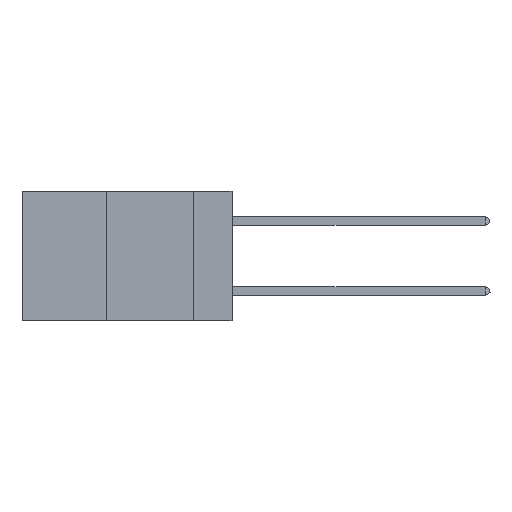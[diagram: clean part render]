
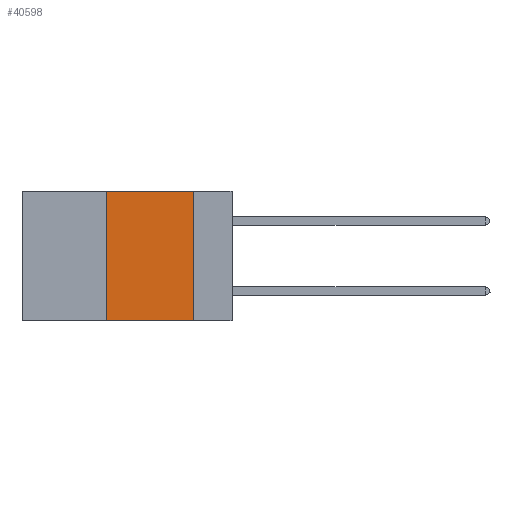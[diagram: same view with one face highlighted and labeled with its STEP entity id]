
A CAD part, left-side view. The second image highlights one B-rep face of the part: STEP entity #40598.
In plain terms, the highlighted planar face has unit normal (-1, 0, 0).
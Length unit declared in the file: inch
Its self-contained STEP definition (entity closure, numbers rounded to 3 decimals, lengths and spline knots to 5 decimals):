
#382 = CARTESIAN_POINT ( 'NONE',  ( 0., 0.36, 0. ) ) ;
#1065 = VECTOR ( 'NONE', #1527, 39.37008 ) ;
#1527 = DIRECTION ( 'NONE',  ( 0., -1., 0. ) ) ;
#1857 = PLANE ( 'NONE',  #9017 ) ;
#2137 = VECTOR ( 'NONE', #36991, 39.37008 ) ;
#2218 = FACE_OUTER_BOUND ( 'NONE', #4220, .T. ) ;
#4220 = EDGE_LOOP ( 'NONE', ( #26346, #16620, #9751, #11718 ) ) ;
#6158 = EDGE_CURVE ( 'NONE', #21618, #41178, #9960, .T. ) ;
#6768 = CARTESIAN_POINT ( 'NONE',  ( 0., 0.6, -0.37 ) ) ;
#8597 = CARTESIAN_POINT ( 'NONE',  ( 0., 0.36, -0.37 ) ) ;
#9017 = AXIS2_PLACEMENT_3D ( 'NONE', #24140, #38296, #34073 ) ;
#9751 = ORIENTED_EDGE ( 'NONE', *, *, #23427, .F. ) ;
#9761 = CARTESIAN_POINT ( 'NONE',  ( 0., 0.36, 0. ) ) ;
#9960 = LINE ( 'NONE', #25116, #1065 ) ;
#11718 = ORIENTED_EDGE ( 'NONE', *, *, #18143, .T. ) ;
#13224 = DIRECTION ( 'NONE',  ( 0., -1., 0. ) ) ;
#16587 = CARTESIAN_POINT ( 'NONE',  ( 0., 0.11, 0. ) ) ;
#16620 = ORIENTED_EDGE ( 'NONE', *, *, #6158, .F. ) ;
#18143 = EDGE_CURVE ( 'NONE', #23199, #40075, #41325, .T. ) ;
#21291 = CARTESIAN_POINT ( 'NONE',  ( 0., 0.11, -0.37 ) ) ;
#21618 = VERTEX_POINT ( 'NONE', #9761 ) ;
#23124 = EDGE_CURVE ( 'NONE', #41178, #40075, #40264, .T. ) ;
#23199 = VERTEX_POINT ( 'NONE', #8597 ) ;
#23427 = EDGE_CURVE ( 'NONE', #23199, #21618, #26120, .T. ) ;
#24140 = CARTESIAN_POINT ( 'NONE',  ( 0., 0.6, 0. ) ) ;
#25116 = CARTESIAN_POINT ( 'NONE',  ( 0., 0.6, 0. ) ) ;
#26120 = LINE ( 'NONE', #382, #2137 ) ;
#26346 = ORIENTED_EDGE ( 'NONE', *, *, #23124, .F. ) ;
#30851 = VECTOR ( 'NONE', #40953, 39.37008 ) ;
#30852 = CARTESIAN_POINT ( 'NONE',  ( 0., 0.11, 0. ) ) ;
#34073 = DIRECTION ( 'NONE',  ( 0., 0., -1. ) ) ;
#36991 = DIRECTION ( 'NONE',  ( 0., 0., 1. ) ) ;
#38296 = DIRECTION ( 'NONE',  ( 1., 0., 0. ) ) ;
#38727 = VECTOR ( 'NONE', #13224, 39.37008 ) ;
#40075 = VERTEX_POINT ( 'NONE', #21291 ) ;
#40264 = LINE ( 'NONE', #30852, #30851 ) ;
#40598 = ADVANCED_FACE ( 'NONE', ( #2218 ), #1857, .F. ) ;
#40953 = DIRECTION ( 'NONE',  ( 0., 0., -1. ) ) ;
#41178 = VERTEX_POINT ( 'NONE', #16587 ) ;
#41325 = LINE ( 'NONE', #6768, #38727 ) ;
